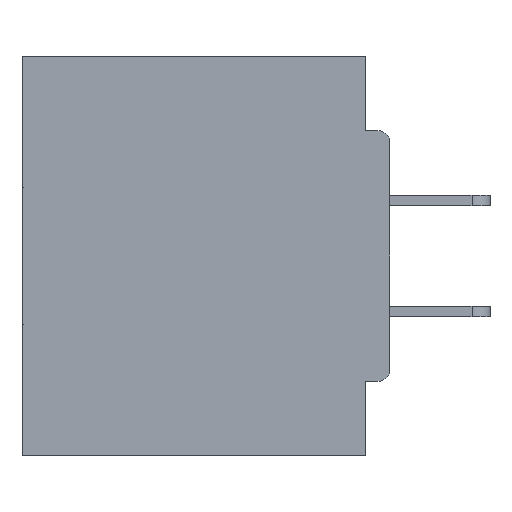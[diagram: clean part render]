
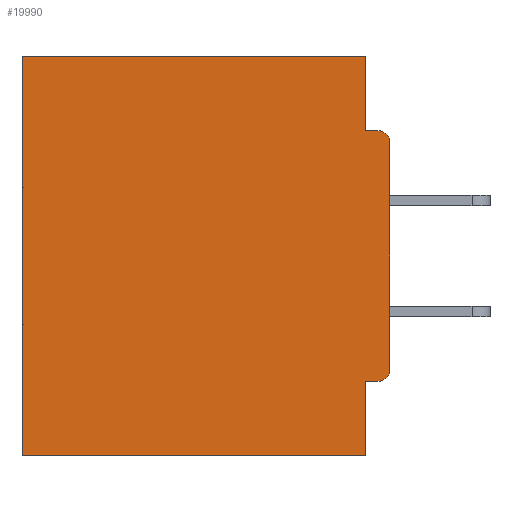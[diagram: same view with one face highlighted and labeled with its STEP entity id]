
A CAD part, left-side view. The second image highlights one B-rep face of the part: STEP entity #19990.
In plain terms, the highlighted planar face has unit normal (-1, 0, 0).
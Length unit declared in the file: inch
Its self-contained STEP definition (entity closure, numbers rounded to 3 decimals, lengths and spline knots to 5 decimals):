
#732 = ORIENTED_EDGE ( 'NONE', *, *, #2938, .F. ) ;
#843 = DIRECTION ( 'NONE',  ( 0., 0., -1. ) ) ;
#881 = CARTESIAN_POINT ( 'NONE',  ( 0.298, 0.031, -0.5 ) ) ;
#1734 = DIRECTION ( 'NONE',  ( 0., 0., -1. ) ) ;
#2818 = EDGE_CURVE ( 'NONE', #4591, #12257, #36136, .T. ) ;
#2938 = EDGE_CURVE ( 'NONE', #33095, #9468, #34677, .T. ) ;
#3002 = ORIENTED_EDGE ( 'NONE', *, *, #22242, .F. ) ;
#4088 = CARTESIAN_POINT ( 'NONE',  ( 0.298, 0., 0. ) ) ;
#4177 = DIRECTION ( 'NONE',  ( -1., 0., 0. ) ) ;
#4255 = VECTOR ( 'NONE', #21597, 39.37008 ) ;
#4591 = VERTEX_POINT ( 'NONE', #8005 ) ;
#4711 = CARTESIAN_POINT ( 'NONE',  ( 0.298, 0.031, -0.4065 ) ) ;
#4725 = LINE ( 'NONE', #34924, #21657 ) ;
#4777 = CARTESIAN_POINT ( 'NONE',  ( 0.298, 0.031, -0.5 ) ) ;
#4845 = EDGE_LOOP ( 'NONE', ( #22708, #8864, #732, #5149, #25483, #40778, #26277, #16490, #31438, #3002 ) ) ;
#5086 = CARTESIAN_POINT ( 'NONE',  ( 0.298, 0.031, 0. ) ) ;
#5149 = ORIENTED_EDGE ( 'NONE', *, *, #6920, .T. ) ;
#5193 = CARTESIAN_POINT ( 'NONE',  ( 0.298, 0., -0.5 ) ) ;
#5237 = AXIS2_PLACEMENT_3D ( 'NONE', #21570, #15453, #18486 ) ;
#6547 = DIRECTION ( 'NONE',  ( 0., -1., 0. ) ) ;
#6920 = EDGE_CURVE ( 'NONE', #33095, #19251, #4725, .T. ) ;
#7039 = CARTESIAN_POINT ( 'NONE',  ( 0.298, 0., -0.4065 ) ) ;
#7132 = VERTEX_POINT ( 'NONE', #881 ) ;
#7287 = DIRECTION ( 'NONE',  ( 0., 0., -1. ) ) ;
#7854 = CARTESIAN_POINT ( 'NONE',  ( 0.298, 0., -0.3915 ) ) ;
#8005 = CARTESIAN_POINT ( 'NONE',  ( 0.298, 0.015, -0.4065 ) ) ;
#8710 = EDGE_CURVE ( 'NONE', #9468, #21983, #11148, .T. ) ;
#8864 = ORIENTED_EDGE ( 'NONE', *, *, #8710, .F. ) ;
#9144 = DIRECTION ( 'NONE',  ( 0., 0., -1. ) ) ;
#9416 = CIRCLE ( 'NONE', #36076, 0.015 ) ;
#9468 = VERTEX_POINT ( 'NONE', #14066 ) ;
#11053 = EDGE_CURVE ( 'NONE', #4591, #40461, #9416, .T. ) ;
#11148 = LINE ( 'NONE', #16554, #22576 ) ;
#11948 = DIRECTION ( 'NONE',  ( -1., 0., 0. ) ) ;
#11971 = LINE ( 'NONE', #34314, #30379 ) ;
#12257 = VERTEX_POINT ( 'NONE', #4711 ) ;
#12265 = AXIS2_PLACEMENT_3D ( 'NONE', #41013, #11948, #21810 ) ;
#14066 = CARTESIAN_POINT ( 'NONE',  ( 0.298, 0.031, -0.0935 ) ) ;
#15184 = LINE ( 'NONE', #5193, #4255 ) ;
#15313 = PLANE ( 'NONE',  #5237 ) ;
#15453 = DIRECTION ( 'NONE',  ( 1., 0., 0. ) ) ;
#15542 = CARTESIAN_POINT ( 'NONE',  ( 0.298, 0.46, -0.5 ) ) ;
#15598 = VERTEX_POINT ( 'NONE', #15542 ) ;
#16490 = ORIENTED_EDGE ( 'NONE', *, *, #2818, .F. ) ;
#16554 = CARTESIAN_POINT ( 'NONE',  ( 0.298, 0., -0.0935 ) ) ;
#18486 = DIRECTION ( 'NONE',  ( 0., 0., -1. ) ) ;
#18808 = VECTOR ( 'NONE', #7287, 39.37008 ) ;
#19251 = VERTEX_POINT ( 'NONE', #19430 ) ;
#19430 = CARTESIAN_POINT ( 'NONE',  ( 0.298, 0.46, 0. ) ) ;
#19990 = ADVANCED_FACE ( 'NONE', ( #25989 ), #15313, .F. ) ;
#21570 = CARTESIAN_POINT ( 'NONE',  ( 0.298, 0., 0. ) ) ;
#21597 = DIRECTION ( 'NONE',  ( 0., 1., 0. ) ) ;
#21657 = VECTOR ( 'NONE', #32146, 39.37008 ) ;
#21810 = DIRECTION ( 'NONE',  ( 0., 0., -1. ) ) ;
#21983 = VERTEX_POINT ( 'NONE', #28576 ) ;
#22242 = EDGE_CURVE ( 'NONE', #28001, #40461, #26791, .T. ) ;
#22576 = VECTOR ( 'NONE', #6547, 39.37008 ) ;
#22708 = ORIENTED_EDGE ( 'NONE', *, *, #30805, .T. ) ;
#23300 = DIRECTION ( 'NONE',  ( 0., 1., 0. ) ) ;
#23839 = CARTESIAN_POINT ( 'NONE',  ( 0.298, 0.031, -0.5 ) ) ;
#24228 = VECTOR ( 'NONE', #1734, 39.37008 ) ;
#25150 = EDGE_CURVE ( 'NONE', #7132, #15598, #15184, .T. ) ;
#25483 = ORIENTED_EDGE ( 'NONE', *, *, #38866, .T. ) ;
#25989 = FACE_OUTER_BOUND ( 'NONE', #4845, .T. ) ;
#26214 = VECTOR ( 'NONE', #23300, 39.37008 ) ;
#26277 = ORIENTED_EDGE ( 'NONE', *, *, #36938, .F. ) ;
#26333 = CARTESIAN_POINT ( 'NONE',  ( 0.298, 0., -0.1085 ) ) ;
#26791 = LINE ( 'NONE', #4088, #18808 ) ;
#28001 = VERTEX_POINT ( 'NONE', #26333 ) ;
#28576 = CARTESIAN_POINT ( 'NONE',  ( 0.298, 0.015, -0.0935 ) ) ;
#30355 = DIRECTION ( 'NONE',  ( 0., 0., -1. ) ) ;
#30379 = VECTOR ( 'NONE', #9144, 39.37008 ) ;
#30805 = EDGE_CURVE ( 'NONE', #28001, #21983, #36559, .T. ) ;
#31438 = ORIENTED_EDGE ( 'NONE', *, *, #11053, .T. ) ;
#32146 = DIRECTION ( 'NONE',  ( 0., 1., 0. ) ) ;
#33095 = VERTEX_POINT ( 'NONE', #5086 ) ;
#34314 = CARTESIAN_POINT ( 'NONE',  ( 0.298, 0.46, 0. ) ) ;
#34677 = LINE ( 'NONE', #23839, #24228 ) ;
#34924 = CARTESIAN_POINT ( 'NONE',  ( 0.298, 0., 0. ) ) ;
#35822 = VECTOR ( 'NONE', #30355, 39.37008 ) ;
#36076 = AXIS2_PLACEMENT_3D ( 'NONE', #39219, #4177, #843 ) ;
#36136 = LINE ( 'NONE', #7039, #26214 ) ;
#36559 = CIRCLE ( 'NONE', #12265, 0.015 ) ;
#36938 = EDGE_CURVE ( 'NONE', #12257, #7132, #39862, .T. ) ;
#38866 = EDGE_CURVE ( 'NONE', #19251, #15598, #11971, .T. ) ;
#39219 = CARTESIAN_POINT ( 'NONE',  ( 0.298, 0.015, -0.3915 ) ) ;
#39862 = LINE ( 'NONE', #4777, #35822 ) ;
#40461 = VERTEX_POINT ( 'NONE', #7854 ) ;
#40778 = ORIENTED_EDGE ( 'NONE', *, *, #25150, .F. ) ;
#41013 = CARTESIAN_POINT ( 'NONE',  ( 0.298, 0.015, -0.1085 ) ) ;
